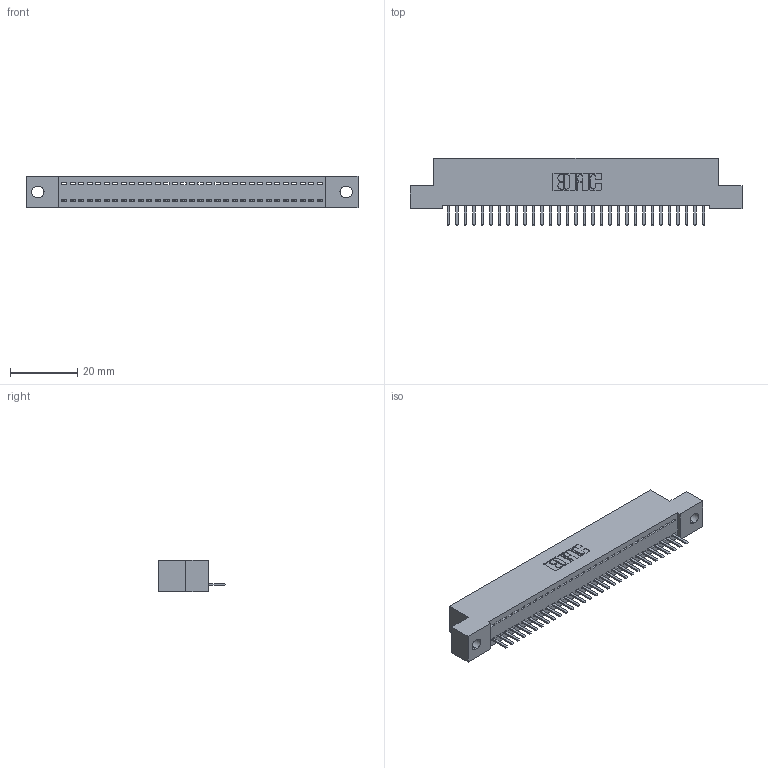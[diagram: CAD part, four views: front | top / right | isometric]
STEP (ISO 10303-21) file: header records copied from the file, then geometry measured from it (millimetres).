
FILE_DESCRIPTION (( 'STEP AP203' ), '1' );
FILE_NAME ('342-031-520-102.STEP', '2018-08-11T16:04:09', ( '' ), ( '' ), 'SwSTEP 2.0', 'SolidWorks 2016', '' );
FILE_SCHEMA (( 'CONFIG_CONTROL_DESIGN' ));
Length unit declared in the file: inch
Products named in the file (3): 345-292-001_345-293-120; 342-031-520-102; 342 Part_.128 Slot
Assembly tree (32 placements, depth 2):
  342-031-520-102
    342 Part_.128 Slot
    345-292-001_345-293-120  x31
Bounding box: 99.06 x 20.02 x 9.4 mm (x, y, z)
Volume: 8503.7 mm3; surface area: 11756.4 mm2
Topology: 32 solids, 32 shells, 2036 faces, 6015 edges, 3926 vertices
Faces by surface type: plane 1434, cylinder 602
Entity records: 20491 total; most frequent: CARTESIAN_POINT 3555, ORIENTED_EDGE 3510, DIRECTION 3009, EDGE_CURVE 1755, LINE 1623, VECTOR 1623, VERTEX_POINT 1166, AXIS2_PLACEMENT_3D 693
